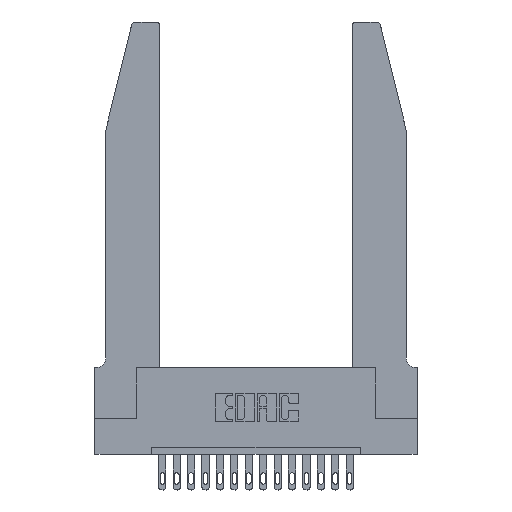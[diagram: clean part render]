
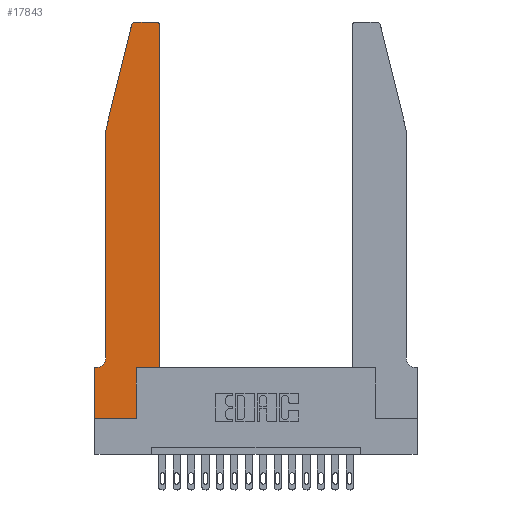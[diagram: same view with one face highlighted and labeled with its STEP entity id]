
A CAD part, top view. The second image highlights one B-rep face of the part: STEP entity #17843.
In plain terms, the highlighted planar face has unit normal (0, 0, 1).
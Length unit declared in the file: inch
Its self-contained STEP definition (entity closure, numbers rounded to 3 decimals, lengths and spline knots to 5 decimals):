
#169 = CARTESIAN_POINT ( 'NONE',  ( 0.2865, 0.35, 0.37 ) ) ;
#391 = DIRECTION ( 'NONE',  ( 1., 0., 0. ) ) ;
#498 = DIRECTION ( 'NONE',  ( 0., 0., 1. ) ) ;
#745 = ORIENTED_EDGE ( 'NONE', *, *, #11778, .T. ) ;
#824 = ORIENTED_EDGE ( 'NONE', *, *, #3113, .T. ) ;
#1103 = VERTEX_POINT ( 'NONE', #12734 ) ;
#1182 = EDGE_CURVE ( 'NONE', #17235, #5215, #17721, .T. ) ;
#1188 = CARTESIAN_POINT ( 'NONE',  ( 0.0755, 2., 0.37 ) ) ;
#1355 = CARTESIAN_POINT ( 'NONE',  ( 0.0755, 0.35, 0.37 ) ) ;
#1954 = VERTEX_POINT ( 'NONE', #9562 ) ;
#2242 = CARTESIAN_POINT ( 'NONE',  ( 0.0055, 0.42, 0.37 ) ) ;
#2367 = EDGE_CURVE ( 'NONE', #12427, #1103, #10491, .T. ) ;
#2613 = VECTOR ( 'NONE', #9892, 39.37008 ) ;
#2838 = CIRCLE ( 'NONE', #5597, 0.07 ) ;
#2893 = VERTEX_POINT ( 'NONE', #3287 ) ;
#2905 = VERTEX_POINT ( 'NONE', #5800 ) ;
#2983 = PLANE ( 'NONE',  #13179 ) ;
#3059 = DIRECTION ( 'NONE',  ( 0., 1., 0. ) ) ;
#3077 = DIRECTION ( 'NONE',  ( 1., 0., 0. ) ) ;
#3113 = EDGE_CURVE ( 'NONE', #2893, #18962, #13002, .T. ) ;
#3233 = ORIENTED_EDGE ( 'NONE', *, *, #15715, .T. ) ;
#3262 = CARTESIAN_POINT ( 'NONE',  ( 0.284, 2.75, 0.37 ) ) ;
#3287 = CARTESIAN_POINT ( 'NONE',  ( 0.2865, 0., 0.37 ) ) ;
#3610 = EDGE_CURVE ( 'NONE', #5215, #2893, #13456, .T. ) ;
#3735 = DIRECTION ( 'NONE',  ( 0., 0., -1. ) ) ;
#3792 = CARTESIAN_POINT ( 'NONE',  ( 0.284, 2.72, 0.37 ) ) ;
#3811 = EDGE_CURVE ( 'NONE', #6815, #2905, #10432, .T. ) ;
#4130 = VECTOR ( 'NONE', #3059, 39.37008 ) ;
#4142 = ORIENTED_EDGE ( 'NONE', *, *, #8276, .T. ) ;
#4231 = DIRECTION ( 'NONE',  ( 0., -1., 0. ) ) ;
#5040 = VECTOR ( 'NONE', #8940, 39.37008 ) ;
#5105 = LINE ( 'NONE', #11673, #6906 ) ;
#5160 = CARTESIAN_POINT ( 'NONE',  ( 0., 0.35, 0.37 ) ) ;
#5215 = VERTEX_POINT ( 'NONE', #15265 ) ;
#5529 = VERTEX_POINT ( 'NONE', #11719 ) ;
#5597 = AXIS2_PLACEMENT_3D ( 'NONE', #2242, #3735, #12578 ) ;
#5800 = CARTESIAN_POINT ( 'NONE',  ( 0.25487, 2.72718, 0.37 ) ) ;
#6137 = CARTESIAN_POINT ( 'NONE',  ( 0., 0.35, 0.37 ) ) ;
#6622 = ORIENTED_EDGE ( 'NONE', *, *, #9117, .T. ) ;
#6815 = VERTEX_POINT ( 'NONE', #3262 ) ;
#6906 = VECTOR ( 'NONE', #3077, 39.37008 ) ;
#6968 = LINE ( 'NONE', #1188, #2613 ) ;
#6969 = ORIENTED_EDGE ( 'NONE', *, *, #3610, .T. ) ;
#6992 = EDGE_CURVE ( 'NONE', #18962, #12427, #5105, .T. ) ;
#7083 = VECTOR ( 'NONE', #14654, 39.37008 ) ;
#7542 = FACE_OUTER_BOUND ( 'NONE', #17925, .T. ) ;
#7624 = CIRCLE ( 'NONE', #8479, 0.03 ) ;
#8213 = ORIENTED_EDGE ( 'NONE', *, *, #16024, .T. ) ;
#8276 = EDGE_CURVE ( 'NONE', #11796, #17235, #15532, .T. ) ;
#8479 = AXIS2_PLACEMENT_3D ( 'NONE', #18068, #13479, #391 ) ;
#8626 = LINE ( 'NONE', #10825, #12730 ) ;
#8693 = CARTESIAN_POINT ( 'NONE',  ( 0.0055, 0.35, 0.37 ) ) ;
#8890 = CARTESIAN_POINT ( 'NONE',  ( 0., 0., 0.37 ) ) ;
#8940 = DIRECTION ( 'NONE',  ( 1., 0., 0. ) ) ;
#9117 = EDGE_CURVE ( 'NONE', #16488, #6815, #8626, .T. ) ;
#9562 = CARTESIAN_POINT ( 'NONE',  ( 0.0755, 2., 0.37 ) ) ;
#9844 = VECTOR ( 'NONE', #4231, 39.37008 ) ;
#9892 = DIRECTION ( 'NONE',  ( 0., -1., 0. ) ) ;
#10410 = CARTESIAN_POINT ( 'NONE',  ( 0.4205, 2.75, 0.37 ) ) ;
#10432 = CIRCLE ( 'NONE', #12106, 0.03 ) ;
#10491 = LINE ( 'NONE', #12452, #15106 ) ;
#10551 = ORIENTED_EDGE ( 'NONE', *, *, #3811, .T. ) ;
#10825 = CARTESIAN_POINT ( 'NONE',  ( 0.2605, 2.75, 0.37 ) ) ;
#10941 = ORIENTED_EDGE ( 'NONE', *, *, #2367, .T. ) ;
#11449 = DIRECTION ( 'NONE',  ( 0., 1., 0. ) ) ;
#11471 = EDGE_CURVE ( 'NONE', #1954, #5529, #6968, .T. ) ;
#11673 = CARTESIAN_POINT ( 'NONE',  ( 0.4505, 0.35, 0.37 ) ) ;
#11719 = CARTESIAN_POINT ( 'NONE',  ( 0.0755, 0.42, 0.37 ) ) ;
#11740 = CARTESIAN_POINT ( 'NONE',  ( 0.2865, 0.35, 0.37 ) ) ;
#11778 = EDGE_CURVE ( 'NONE', #2905, #1954, #12317, .T. ) ;
#11796 = VERTEX_POINT ( 'NONE', #8693 ) ;
#12106 = AXIS2_PLACEMENT_3D ( 'NONE', #3792, #18388, #15448 ) ;
#12317 = LINE ( 'NONE', #13665, #16924 ) ;
#12427 = VERTEX_POINT ( 'NONE', #16909 ) ;
#12452 = CARTESIAN_POINT ( 'NONE',  ( 0.4505, 0.35, 0.37 ) ) ;
#12578 = DIRECTION ( 'NONE',  ( -1., 0., 0. ) ) ;
#12730 = VECTOR ( 'NONE', #15010, 39.37008 ) ;
#12734 = CARTESIAN_POINT ( 'NONE',  ( 0.4505, 2.72, 0.37 ) ) ;
#13002 = LINE ( 'NONE', #169, #4130 ) ;
#13039 = ORIENTED_EDGE ( 'NONE', *, *, #6992, .T. ) ;
#13179 = AXIS2_PLACEMENT_3D ( 'NONE', #6137, #498, #17854 ) ;
#13456 = LINE ( 'NONE', #17909, #5040 ) ;
#13479 = DIRECTION ( 'NONE',  ( 0., 0., 1. ) ) ;
#13665 = CARTESIAN_POINT ( 'NONE',  ( 0.0755, 2., 0.37 ) ) ;
#14654 = DIRECTION ( 'NONE',  ( -1., 0., 0. ) ) ;
#14761 = ORIENTED_EDGE ( 'NONE', *, *, #11471, .T. ) ;
#15010 = DIRECTION ( 'NONE',  ( -1., 0., 0. ) ) ;
#15106 = VECTOR ( 'NONE', #11449, 39.37008 ) ;
#15265 = CARTESIAN_POINT ( 'NONE',  ( 0., 0., 0.37 ) ) ;
#15448 = DIRECTION ( 'NONE',  ( 1., 0., 0. ) ) ;
#15532 = LINE ( 'NONE', #1355, #7083 ) ;
#15715 = EDGE_CURVE ( 'NONE', #5529, #11796, #2838, .T. ) ;
#15777 = ORIENTED_EDGE ( 'NONE', *, *, #1182, .T. ) ;
#16024 = EDGE_CURVE ( 'NONE', #1103, #16488, #7624, .T. ) ;
#16488 = VERTEX_POINT ( 'NONE', #10410 ) ;
#16826 = DIRECTION ( 'NONE',  ( -0.239, -0.971, 0. ) ) ;
#16909 = CARTESIAN_POINT ( 'NONE',  ( 0.4505, 0.35, 0.37 ) ) ;
#16924 = VECTOR ( 'NONE', #16826, 39.37008 ) ;
#17235 = VERTEX_POINT ( 'NONE', #5160 ) ;
#17721 = LINE ( 'NONE', #8890, #9844 ) ;
#17843 = ADVANCED_FACE ( 'NONE', ( #7542 ), #2983, .T. ) ;
#17854 = DIRECTION ( 'NONE',  ( 1., 0., 0. ) ) ;
#17909 = CARTESIAN_POINT ( 'NONE',  ( 0., 0., 0.37 ) ) ;
#17925 = EDGE_LOOP ( 'NONE', ( #6622, #10551, #745, #14761, #3233, #4142, #15777, #6969, #824, #13039, #10941, #8213 ) ) ;
#18068 = CARTESIAN_POINT ( 'NONE',  ( 0.4205, 2.72, 0.37 ) ) ;
#18388 = DIRECTION ( 'NONE',  ( 0., 0., 1. ) ) ;
#18962 = VERTEX_POINT ( 'NONE', #11740 ) ;
